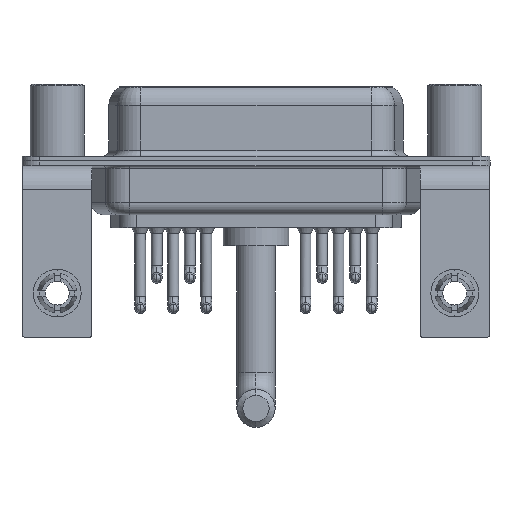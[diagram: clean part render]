
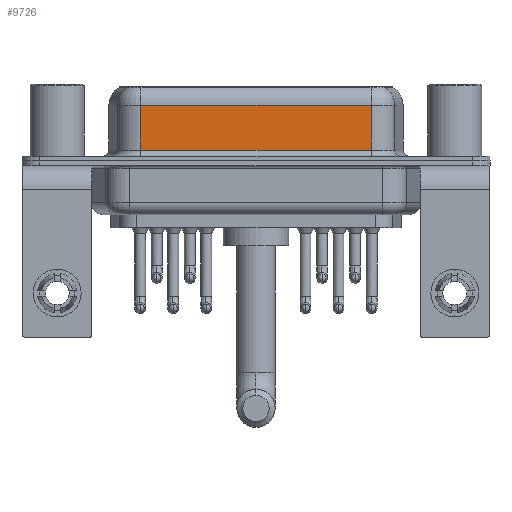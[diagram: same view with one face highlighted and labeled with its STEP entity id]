
A CAD part, front view. The second image highlights one B-rep face of the part: STEP entity #9726.
In plain terms, the highlighted planar face has unit normal (0, -1, 0).
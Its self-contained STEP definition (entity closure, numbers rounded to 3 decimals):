
#245 = CARTESIAN_POINT ( 'NONE',  ( 7.013, -3.95, 0.9 ) ) ;
#485 = VECTOR ( 'NONE', #20815, 1000. ) ;
#1230 = VERTEX_POINT ( 'NONE', #8460 ) ;
#1469 = EDGE_LOOP ( 'NONE', ( #17255, #19353, #2979, #19817 ) ) ;
#2979 = ORIENTED_EDGE ( 'NONE', *, *, #15274, .T. ) ;
#3539 = DIRECTION ( 'NONE',  ( 0., 0., 1. ) ) ;
#3945 = VECTOR ( 'NONE', #4584, 1000. ) ;
#4574 = AXIS2_PLACEMENT_3D ( 'NONE', #10235, #13687, #3539 ) ;
#4584 = DIRECTION ( 'NONE',  ( 0., 0., -1. ) ) ;
#4909 = FACE_OUTER_BOUND ( 'NONE', #1469, .T. ) ;
#5438 = VECTOR ( 'NONE', #6445, 1000. ) ;
#5821 = CARTESIAN_POINT ( 'NONE',  ( 26.287, -3.95, 0.9 ) ) ;
#6073 = CARTESIAN_POINT ( 'NONE',  ( 26.287, -3.95, 4.65 ) ) ;
#6445 = DIRECTION ( 'NONE',  ( 0., 0., -1. ) ) ;
#7847 = CARTESIAN_POINT ( 'NONE',  ( 26.287, -3.95, 0.9 ) ) ;
#7945 = LINE ( 'NONE', #18667, #3945 ) ;
#8460 = CARTESIAN_POINT ( 'NONE',  ( 26.287, -3.95, 4.65 ) ) ;
#8704 = EDGE_CURVE ( 'NONE', #1230, #18198, #20697, .T. ) ;
#9726 = ADVANCED_FACE ( 'NONE', ( #4909 ), #17629, .F. ) ;
#9915 = CARTESIAN_POINT ( 'NONE',  ( 26.287, -3.95, 6.4 ) ) ;
#9953 = VERTEX_POINT ( 'NONE', #5821 ) ;
#10235 = CARTESIAN_POINT ( 'NONE',  ( 26.287, -3.95, 6.4 ) ) ;
#11203 = DIRECTION ( 'NONE',  ( 1., 0., 0. ) ) ;
#12894 = CARTESIAN_POINT ( 'NONE',  ( 7.013, -3.95, 4.65 ) ) ;
#13687 = DIRECTION ( 'NONE',  ( 0., 1., 0. ) ) ;
#15274 = EDGE_CURVE ( 'NONE', #18198, #19671, #7945, .T. ) ;
#16222 = EDGE_CURVE ( 'NONE', #19671, #9953, #18121, .T. ) ;
#16415 = EDGE_CURVE ( 'NONE', #1230, #9953, #18457, .T. ) ;
#17255 = ORIENTED_EDGE ( 'NONE', *, *, #16415, .F. ) ;
#17629 = PLANE ( 'NONE',  #4574 ) ;
#18121 = LINE ( 'NONE', #7847, #20178 ) ;
#18198 = VERTEX_POINT ( 'NONE', #12894 ) ;
#18457 = LINE ( 'NONE', #9915, #5438 ) ;
#18667 = CARTESIAN_POINT ( 'NONE',  ( 7.013, -3.95, 6.4 ) ) ;
#19353 = ORIENTED_EDGE ( 'NONE', *, *, #8704, .T. ) ;
#19671 = VERTEX_POINT ( 'NONE', #245 ) ;
#19817 = ORIENTED_EDGE ( 'NONE', *, *, #16222, .T. ) ;
#20178 = VECTOR ( 'NONE', #11203, 1000. ) ;
#20697 = LINE ( 'NONE', #6073, #485 ) ;
#20815 = DIRECTION ( 'NONE',  ( -1., 0., 0. ) ) ;
